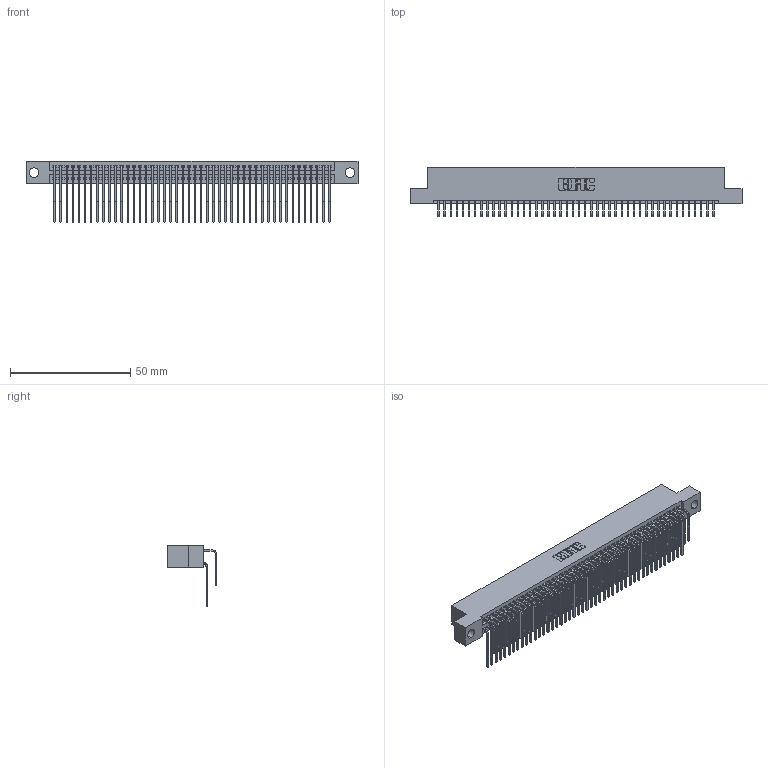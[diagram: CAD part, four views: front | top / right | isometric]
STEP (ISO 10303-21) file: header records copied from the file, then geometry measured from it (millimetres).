
FILE_DESCRIPTION (( 'STEP AP203' ), '1' );
FILE_NAME ('395-092-559-204.STEP', '2021-06-17T11:04:31', ( '' ), ( '' ), 'SwSTEP 2.0', 'SolidWorks 2020', '' );
FILE_SCHEMA (( 'CONFIG_CONTROL_DESIGN' ));
Length unit declared in the file: inch
Products named in the file (4): 345-292-001_558 559 Tail - 1; 345 Part_Flush Mounting Lugs - 0.156 Dia-TI; 345-292-001_559 Tail - 2; 395-092-559-204
Assembly tree (93 placements, depth 2):
  395-092-559-204
    345 Part_Flush Mounting Lugs - 0.156 Dia-TI
    345-292-001_558 559 Tail - 1  x46
    345-292-001_559 Tail - 2  x46
Bounding box: 138.05 x 20.56 x 25.53 mm (x, y, z)
Volume: 13872.1 mm3; surface area: 22930 mm2
Topology: 93 solids, 93 shells, 4924 faces, 14637 edges, 9634 vertices
Faces by surface type: plane 3314, cylinder 1610
Entity records: 37625 total; most frequent: CARTESIAN_POINT 6353, ORIENTED_EDGE 6234, DIRECTION 5569, EDGE_CURVE 3117, VECTOR 2761, LINE 2761, VERTEX_POINT 2074, AXIS2_PLACEMENT_3D 1404
